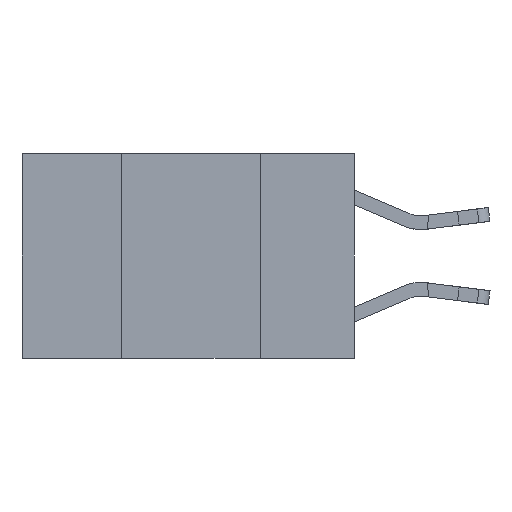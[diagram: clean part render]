
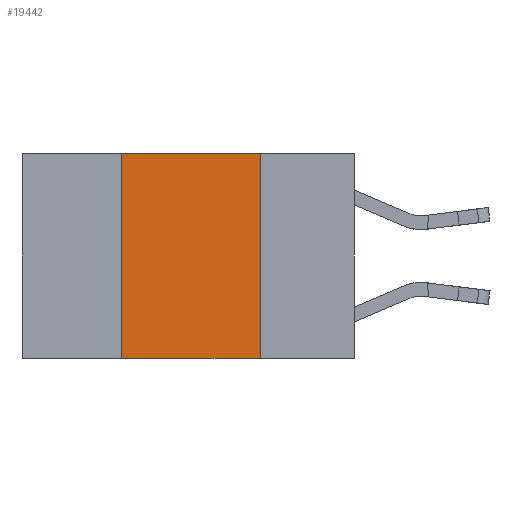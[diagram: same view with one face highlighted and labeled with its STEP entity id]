
A CAD part, left-side view. The second image highlights one B-rep face of the part: STEP entity #19442.
In plain terms, the highlighted planar face has unit normal (-1, 0, 0).
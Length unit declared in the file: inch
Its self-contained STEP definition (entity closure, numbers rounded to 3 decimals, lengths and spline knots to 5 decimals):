
#958 = CARTESIAN_POINT ( 'NONE',  ( 0., 0.6, 0. ) ) ;
#964 = VERTEX_POINT ( 'NONE', #2696 ) ;
#1118 = VECTOR ( 'NONE', #22586, 39.37008 ) ;
#1524 = DIRECTION ( 'NONE',  ( 1., 0., 0. ) ) ;
#1700 = VERTEX_POINT ( 'NONE', #11687 ) ;
#1838 = EDGE_CURVE ( 'NONE', #1700, #3213, #22291, .T. ) ;
#2696 = CARTESIAN_POINT ( 'NONE',  ( 0., 0.17, 0. ) ) ;
#2699 = ORIENTED_EDGE ( 'NONE', *, *, #1838, .F. ) ;
#3213 = VERTEX_POINT ( 'NONE', #14322 ) ;
#4766 = EDGE_LOOP ( 'NONE', ( #9544, #15750, #2699, #5890 ) ) ;
#5030 = LINE ( 'NONE', #20271, #18576 ) ;
#5890 = ORIENTED_EDGE ( 'NONE', *, *, #16657, .T. ) ;
#6806 = CARTESIAN_POINT ( 'NONE',  ( 0., 0.42, 0. ) ) ;
#7353 = DIRECTION ( 'NONE',  ( 0., -1., 0. ) ) ;
#8207 = VERTEX_POINT ( 'NONE', #8948 ) ;
#8948 = CARTESIAN_POINT ( 'NONE',  ( 0., 0.17, -0.37 ) ) ;
#9544 = ORIENTED_EDGE ( 'NONE', *, *, #13069, .F. ) ;
#9623 = CARTESIAN_POINT ( 'NONE',  ( 0., 0.17, 0. ) ) ;
#9769 = VECTOR ( 'NONE', #11877, 39.37008 ) ;
#9916 = EDGE_CURVE ( 'NONE', #3213, #964, #14147, .T. ) ;
#10179 = LINE ( 'NONE', #9623, #1118 ) ;
#11687 = CARTESIAN_POINT ( 'NONE',  ( 0., 0.42, -0.37 ) ) ;
#11877 = DIRECTION ( 'NONE',  ( 0., -1., 0. ) ) ;
#12469 = CARTESIAN_POINT ( 'NONE',  ( 0., 0.6, 0. ) ) ;
#13069 = EDGE_CURVE ( 'NONE', #964, #8207, #10179, .T. ) ;
#13611 = VECTOR ( 'NONE', #21568, 39.37008 ) ;
#14147 = LINE ( 'NONE', #958, #9769 ) ;
#14322 = CARTESIAN_POINT ( 'NONE',  ( 0., 0.42, 0. ) ) ;
#14340 = DIRECTION ( 'NONE',  ( 0., 0., -1. ) ) ;
#15750 = ORIENTED_EDGE ( 'NONE', *, *, #9916, .F. ) ;
#16657 = EDGE_CURVE ( 'NONE', #1700, #8207, #5030, .T. ) ;
#18035 = AXIS2_PLACEMENT_3D ( 'NONE', #12469, #1524, #14340 ) ;
#18189 = FACE_OUTER_BOUND ( 'NONE', #4766, .T. ) ;
#18576 = VECTOR ( 'NONE', #7353, 39.37008 ) ;
#19442 = ADVANCED_FACE ( 'NONE', ( #18189 ), #19840, .F. ) ;
#19840 = PLANE ( 'NONE',  #18035 ) ;
#20271 = CARTESIAN_POINT ( 'NONE',  ( 0., 0.6, -0.37 ) ) ;
#21568 = DIRECTION ( 'NONE',  ( 0., 0., 1. ) ) ;
#22291 = LINE ( 'NONE', #6806, #13611 ) ;
#22586 = DIRECTION ( 'NONE',  ( 0., 0., -1. ) ) ;
